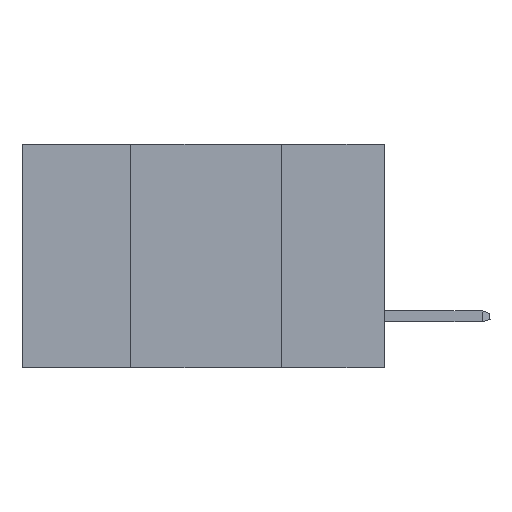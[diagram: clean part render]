
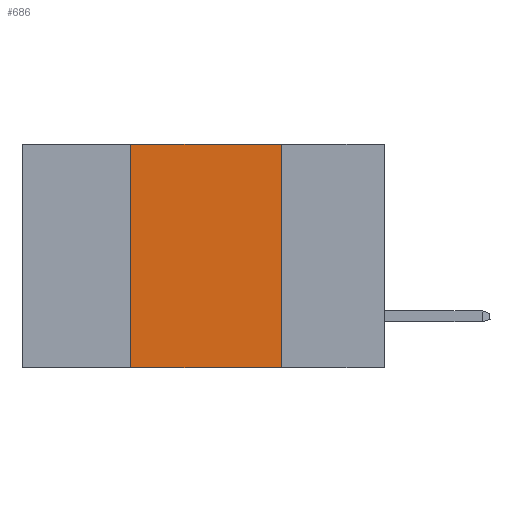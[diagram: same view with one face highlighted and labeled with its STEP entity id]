
A CAD part, left-side view. The second image highlights one B-rep face of the part: STEP entity #686.
In plain terms, the highlighted planar face has unit normal (-1, 0, 0).
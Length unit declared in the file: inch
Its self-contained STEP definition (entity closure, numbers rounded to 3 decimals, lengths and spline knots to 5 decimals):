
#686 = ADVANCED_FACE ( 'NONE', ( #20969 ), #7351, .F. ) ;
#1465 = EDGE_LOOP ( 'NONE', ( #2488, #6870, #11393, #5756 ) ) ;
#1583 = VECTOR ( 'NONE', #15594, 39.37008 ) ;
#1745 = AXIS2_PLACEMENT_3D ( 'NONE', #27248, #22921, #13899 ) ;
#1836 = DIRECTION ( 'NONE',  ( 0., 0., 1. ) ) ;
#2158 = CARTESIAN_POINT ( 'NONE',  ( 0., 0.42, 0. ) ) ;
#2164 = VECTOR ( 'NONE', #3945, 39.37008 ) ;
#2488 = ORIENTED_EDGE ( 'NONE', *, *, #17192, .F. ) ;
#2836 = CARTESIAN_POINT ( 'NONE',  ( 0., 0.17, -0.37 ) ) ;
#3871 = DIRECTION ( 'NONE',  ( 0., -1., 0. ) ) ;
#3945 = DIRECTION ( 'NONE',  ( 0., -1., 0. ) ) ;
#4498 = CARTESIAN_POINT ( 'NONE',  ( 0., 0.17, 0. ) ) ;
#5756 = ORIENTED_EDGE ( 'NONE', *, *, #23898, .T. ) ;
#6870 = ORIENTED_EDGE ( 'NONE', *, *, #11709, .F. ) ;
#7283 = VERTEX_POINT ( 'NONE', #2836 ) ;
#7351 = PLANE ( 'NONE',  #1745 ) ;
#8342 = EDGE_CURVE ( 'NONE', #27206, #13465, #14278, .T. ) ;
#10707 = CARTESIAN_POINT ( 'NONE',  ( 0., 0.17, 0. ) ) ;
#11393 = ORIENTED_EDGE ( 'NONE', *, *, #8342, .F. ) ;
#11709 = EDGE_CURVE ( 'NONE', #13465, #28058, #25193, .T. ) ;
#13465 = VERTEX_POINT ( 'NONE', #2158 ) ;
#13899 = DIRECTION ( 'NONE',  ( 0., 0., -1. ) ) ;
#14278 = LINE ( 'NONE', #15177, #27876 ) ;
#15177 = CARTESIAN_POINT ( 'NONE',  ( 0., 0.42, 0. ) ) ;
#15594 = DIRECTION ( 'NONE',  ( 0., 0., -1. ) ) ;
#17192 = EDGE_CURVE ( 'NONE', #28058, #7283, #21126, .T. ) ;
#19716 = CARTESIAN_POINT ( 'NONE',  ( 0., 0.42, -0.37 ) ) ;
#20969 = FACE_OUTER_BOUND ( 'NONE', #1465, .T. ) ;
#21126 = LINE ( 'NONE', #4498, #1583 ) ;
#21492 = VECTOR ( 'NONE', #3871, 39.37008 ) ;
#22921 = DIRECTION ( 'NONE',  ( 1., 0., 0. ) ) ;
#23847 = CARTESIAN_POINT ( 'NONE',  ( 0., 0.6, -0.37 ) ) ;
#23898 = EDGE_CURVE ( 'NONE', #27206, #7283, #27443, .T. ) ;
#25193 = LINE ( 'NONE', #28457, #2164 ) ;
#27206 = VERTEX_POINT ( 'NONE', #19716 ) ;
#27248 = CARTESIAN_POINT ( 'NONE',  ( 0., 0.6, 0. ) ) ;
#27443 = LINE ( 'NONE', #23847, #21492 ) ;
#27876 = VECTOR ( 'NONE', #1836, 39.37008 ) ;
#28058 = VERTEX_POINT ( 'NONE', #10707 ) ;
#28457 = CARTESIAN_POINT ( 'NONE',  ( 0., 0.6, 0. ) ) ;
